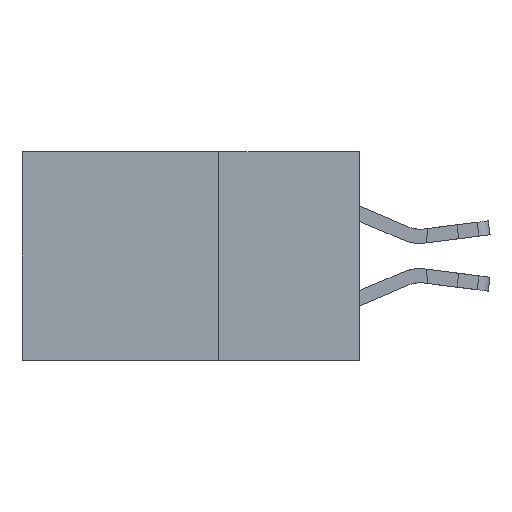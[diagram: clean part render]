
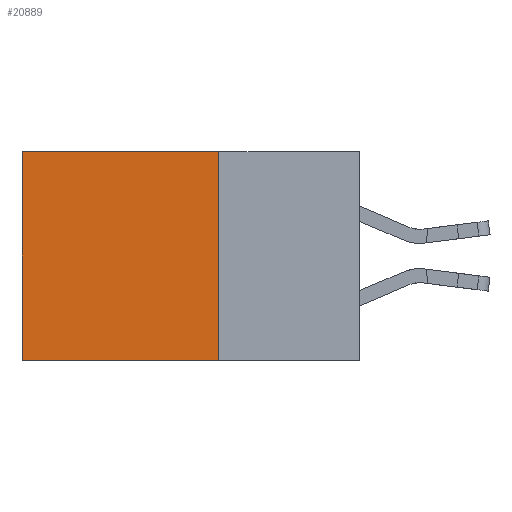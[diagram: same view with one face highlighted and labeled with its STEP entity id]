
A CAD part, left-side view. The second image highlights one B-rep face of the part: STEP entity #20889.
In plain terms, the highlighted planar face has unit normal (-1, 0, 0).
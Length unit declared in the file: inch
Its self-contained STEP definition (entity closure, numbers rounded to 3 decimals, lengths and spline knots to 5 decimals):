
#16 = EDGE_CURVE ( 'NONE', #9463, #5713, #13330, .T. ) ;
#714 = CARTESIAN_POINT ( 'NONE',  ( 0.2875, 0.6, 0. ) ) ;
#896 = DIRECTION ( 'NONE',  ( 0., 0., -1. ) ) ;
#1728 = ORIENTED_EDGE ( 'NONE', *, *, #14190, .T. ) ;
#1971 = DIRECTION ( 'NONE',  ( 0., 0., -1. ) ) ;
#3967 = VECTOR ( 'NONE', #16582, 39.37008 ) ;
#4075 = EDGE_LOOP ( 'NONE', ( #9495, #17595, #14695, #1728 ) ) ;
#5713 = VERTEX_POINT ( 'NONE', #10323 ) ;
#6803 = EDGE_CURVE ( 'NONE', #12982, #9463, #7139, .T. ) ;
#7139 = LINE ( 'NONE', #12393, #9389 ) ;
#7567 = CARTESIAN_POINT ( 'NONE',  ( 0.2875, 0.25, 0. ) ) ;
#7654 = LINE ( 'NONE', #11423, #3967 ) ;
#9122 = EDGE_CURVE ( 'NONE', #18826, #5713, #7654, .T. ) ;
#9389 = VECTOR ( 'NONE', #1971, 39.37008 ) ;
#9463 = VERTEX_POINT ( 'NONE', #17612 ) ;
#9495 = ORIENTED_EDGE ( 'NONE', *, *, #9122, .T. ) ;
#9513 = DIRECTION ( 'NONE',  ( 1., 0., 0. ) ) ;
#10323 = CARTESIAN_POINT ( 'NONE',  ( 0.2875, 0.6, -0.37 ) ) ;
#11396 = VECTOR ( 'NONE', #13923, 39.37008 ) ;
#11423 = CARTESIAN_POINT ( 'NONE',  ( 0.2875, 0.6, 0. ) ) ;
#12393 = CARTESIAN_POINT ( 'NONE',  ( 0.2875, 0.25, 0. ) ) ;
#12982 = VERTEX_POINT ( 'NONE', #19686 ) ;
#13330 = LINE ( 'NONE', #20014, #22280 ) ;
#13923 = DIRECTION ( 'NONE',  ( 0., 1., 0. ) ) ;
#14190 = EDGE_CURVE ( 'NONE', #12982, #18826, #15653, .T. ) ;
#14695 = ORIENTED_EDGE ( 'NONE', *, *, #6803, .F. ) ;
#15653 = LINE ( 'NONE', #15758, #11396 ) ;
#15758 = CARTESIAN_POINT ( 'NONE',  ( 0.2875, 0.25, 0. ) ) ;
#16582 = DIRECTION ( 'NONE',  ( 0., 0., -1. ) ) ;
#17009 = DIRECTION ( 'NONE',  ( 0., 1., 0. ) ) ;
#17595 = ORIENTED_EDGE ( 'NONE', *, *, #16, .F. ) ;
#17612 = CARTESIAN_POINT ( 'NONE',  ( 0.2875, 0.25, -0.37 ) ) ;
#17667 = PLANE ( 'NONE',  #22520 ) ;
#18826 = VERTEX_POINT ( 'NONE', #714 ) ;
#19400 = FACE_OUTER_BOUND ( 'NONE', #4075, .T. ) ;
#19686 = CARTESIAN_POINT ( 'NONE',  ( 0.2875, 0.25, 0. ) ) ;
#20014 = CARTESIAN_POINT ( 'NONE',  ( 0.2875, 0.25, -0.37 ) ) ;
#20889 = ADVANCED_FACE ( 'NONE', ( #19400 ), #17667, .F. ) ;
#22280 = VECTOR ( 'NONE', #17009, 39.37008 ) ;
#22520 = AXIS2_PLACEMENT_3D ( 'NONE', #7567, #9513, #896 ) ;
